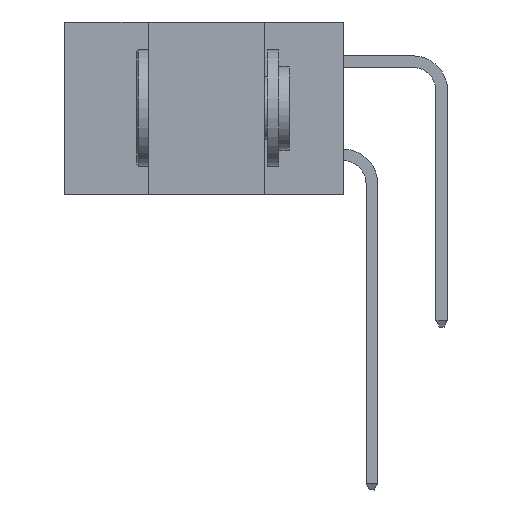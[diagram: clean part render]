
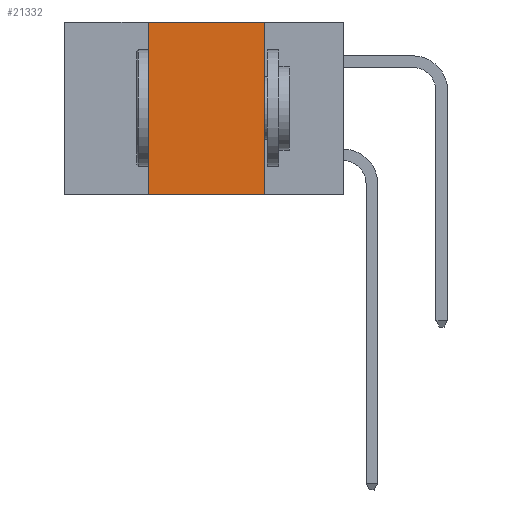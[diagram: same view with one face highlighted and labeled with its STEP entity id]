
A CAD part, left-side view. The second image highlights one B-rep face of the part: STEP entity #21332.
In plain terms, the highlighted planar face has unit normal (-1, 0, 0).
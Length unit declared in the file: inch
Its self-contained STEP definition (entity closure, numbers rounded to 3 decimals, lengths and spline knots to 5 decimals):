
#2717 = ORIENTED_EDGE ( 'NONE', *, *, #19265, .F. ) ;
#2744 = EDGE_CURVE ( 'NONE', #13316, #7763, #3588, .T. ) ;
#2853 = ORIENTED_EDGE ( 'NONE', *, *, #25757, .F. ) ;
#3588 = LINE ( 'NONE', #12141, #10993 ) ;
#5234 = CARTESIAN_POINT ( 'NONE',  ( 0., 0.42, -0.37 ) ) ;
#5687 = VERTEX_POINT ( 'NONE', #23016 ) ;
#6398 = CARTESIAN_POINT ( 'NONE',  ( 0., 0.42, -0.37 ) ) ;
#6603 = LINE ( 'NONE', #26280, #20768 ) ;
#6915 = CARTESIAN_POINT ( 'NONE',  ( 0., 0.17, -0.37 ) ) ;
#7026 = VECTOR ( 'NONE', #15213, 39.37008 ) ;
#7517 = LINE ( 'NONE', #18636, #9405 ) ;
#7664 = DIRECTION ( 'NONE',  ( 0., -1., 0. ) ) ;
#7763 = VERTEX_POINT ( 'NONE', #6915 ) ;
#9405 = VECTOR ( 'NONE', #7664, 39.37008 ) ;
#10178 = FACE_OUTER_BOUND ( 'NONE', #13568, .T. ) ;
#10949 = DIRECTION ( 'NONE',  ( 0., 0., -1. ) ) ;
#10993 = VECTOR ( 'NONE', #16890, 39.37008 ) ;
#12141 = CARTESIAN_POINT ( 'NONE',  ( 0., 0.6, -0.37 ) ) ;
#13316 = VERTEX_POINT ( 'NONE', #5234 ) ;
#13568 = EDGE_LOOP ( 'NONE', ( #2853, #2717, #18759, #27850 ) ) ;
#14089 = CARTESIAN_POINT ( 'NONE',  ( 0., 0.6, 0. ) ) ;
#15213 = DIRECTION ( 'NONE',  ( 0., 0., 1. ) ) ;
#16890 = DIRECTION ( 'NONE',  ( 0., -1., 0. ) ) ;
#17770 = AXIS2_PLACEMENT_3D ( 'NONE', #14089, #25222, #20593 ) ;
#18636 = CARTESIAN_POINT ( 'NONE',  ( 0., 0.6, 0. ) ) ;
#18759 = ORIENTED_EDGE ( 'NONE', *, *, #28119, .F. ) ;
#19265 = EDGE_CURVE ( 'NONE', #5687, #21500, #7517, .T. ) ;
#20593 = DIRECTION ( 'NONE',  ( 0., 0., -1. ) ) ;
#20768 = VECTOR ( 'NONE', #10949, 39.37008 ) ;
#21332 = ADVANCED_FACE ( 'NONE', ( #10178 ), #25662, .F. ) ;
#21500 = VERTEX_POINT ( 'NONE', #26229 ) ;
#23016 = CARTESIAN_POINT ( 'NONE',  ( 0., 0.42, 0. ) ) ;
#25222 = DIRECTION ( 'NONE',  ( 1., 0., 0. ) ) ;
#25662 = PLANE ( 'NONE',  #17770 ) ;
#25757 = EDGE_CURVE ( 'NONE', #21500, #7763, #6603, .T. ) ;
#26225 = LINE ( 'NONE', #6398, #7026 ) ;
#26229 = CARTESIAN_POINT ( 'NONE',  ( 0., 0.17, 0. ) ) ;
#26280 = CARTESIAN_POINT ( 'NONE',  ( 0., 0.17, -0.37 ) ) ;
#27850 = ORIENTED_EDGE ( 'NONE', *, *, #2744, .T. ) ;
#28119 = EDGE_CURVE ( 'NONE', #13316, #5687, #26225, .T. ) ;
